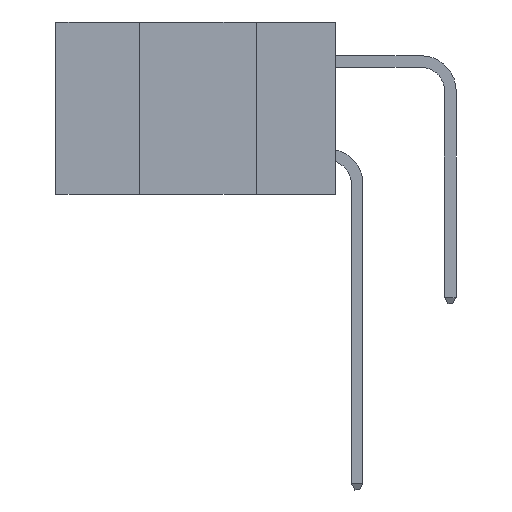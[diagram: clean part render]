
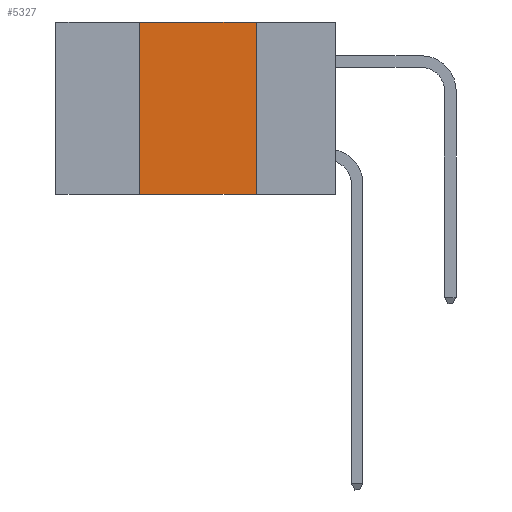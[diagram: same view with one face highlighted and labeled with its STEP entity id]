
A CAD part, left-side view. The second image highlights one B-rep face of the part: STEP entity #5327.
In plain terms, the highlighted planar face has unit normal (-1, 0, 0).
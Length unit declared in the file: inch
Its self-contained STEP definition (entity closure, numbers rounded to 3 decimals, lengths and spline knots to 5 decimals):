
#543 = VERTEX_POINT ( 'NONE', #18567 ) ;
#1604 = CARTESIAN_POINT ( 'NONE',  ( 0., 0.6, 0. ) ) ;
#1932 = DIRECTION ( 'NONE',  ( 0., -1., 0. ) ) ;
#2129 = VERTEX_POINT ( 'NONE', #11722 ) ;
#2306 = VECTOR ( 'NONE', #18248, 39.37008 ) ;
#2317 = DIRECTION ( 'NONE',  ( 0., 0., -1. ) ) ;
#3649 = EDGE_LOOP ( 'NONE', ( #4017, #10458, #7328, #14821 ) ) ;
#4017 = ORIENTED_EDGE ( 'NONE', *, *, #16480, .F. ) ;
#5225 = VECTOR ( 'NONE', #12349, 39.37008 ) ;
#5327 = ADVANCED_FACE ( 'NONE', ( #7627 ), #15715, .F. ) ;
#5350 = CARTESIAN_POINT ( 'NONE',  ( 0., 0.42, 0. ) ) ;
#6338 = EDGE_CURVE ( 'NONE', #13059, #12895, #11090, .T. ) ;
#7328 = ORIENTED_EDGE ( 'NONE', *, *, #17141, .F. ) ;
#7600 = CARTESIAN_POINT ( 'NONE',  ( 0., 0.42, -0.37 ) ) ;
#7627 = FACE_OUTER_BOUND ( 'NONE', #3649, .T. ) ;
#8183 = EDGE_CURVE ( 'NONE', #2129, #543, #9871, .T. ) ;
#9726 = AXIS2_PLACEMENT_3D ( 'NONE', #17018, #11097, #2317 ) ;
#9871 = LINE ( 'NONE', #1604, #17318 ) ;
#10046 = VECTOR ( 'NONE', #14083, 39.37008 ) ;
#10316 = LINE ( 'NONE', #17053, #5225 ) ;
#10458 = ORIENTED_EDGE ( 'NONE', *, *, #8183, .F. ) ;
#11090 = LINE ( 'NONE', #11547, #2306 ) ;
#11097 = DIRECTION ( 'NONE',  ( 1., 0., 0. ) ) ;
#11459 = LINE ( 'NONE', #5350, #10046 ) ;
#11547 = CARTESIAN_POINT ( 'NONE',  ( 0., 0.6, -0.37 ) ) ;
#11722 = CARTESIAN_POINT ( 'NONE',  ( 0., 0.42, 0. ) ) ;
#12349 = DIRECTION ( 'NONE',  ( 0., 0., -1. ) ) ;
#12895 = VERTEX_POINT ( 'NONE', #16124 ) ;
#13059 = VERTEX_POINT ( 'NONE', #7600 ) ;
#14083 = DIRECTION ( 'NONE',  ( 0., 0., 1. ) ) ;
#14821 = ORIENTED_EDGE ( 'NONE', *, *, #6338, .T. ) ;
#15715 = PLANE ( 'NONE',  #9726 ) ;
#16124 = CARTESIAN_POINT ( 'NONE',  ( 0., 0.17, -0.37 ) ) ;
#16480 = EDGE_CURVE ( 'NONE', #543, #12895, #10316, .T. ) ;
#17018 = CARTESIAN_POINT ( 'NONE',  ( 0., 0.6, 0. ) ) ;
#17053 = CARTESIAN_POINT ( 'NONE',  ( 0., 0.17, 0. ) ) ;
#17141 = EDGE_CURVE ( 'NONE', #13059, #2129, #11459, .T. ) ;
#17318 = VECTOR ( 'NONE', #1932, 39.37008 ) ;
#18248 = DIRECTION ( 'NONE',  ( 0., -1., 0. ) ) ;
#18567 = CARTESIAN_POINT ( 'NONE',  ( 0., 0.17, 0. ) ) ;
